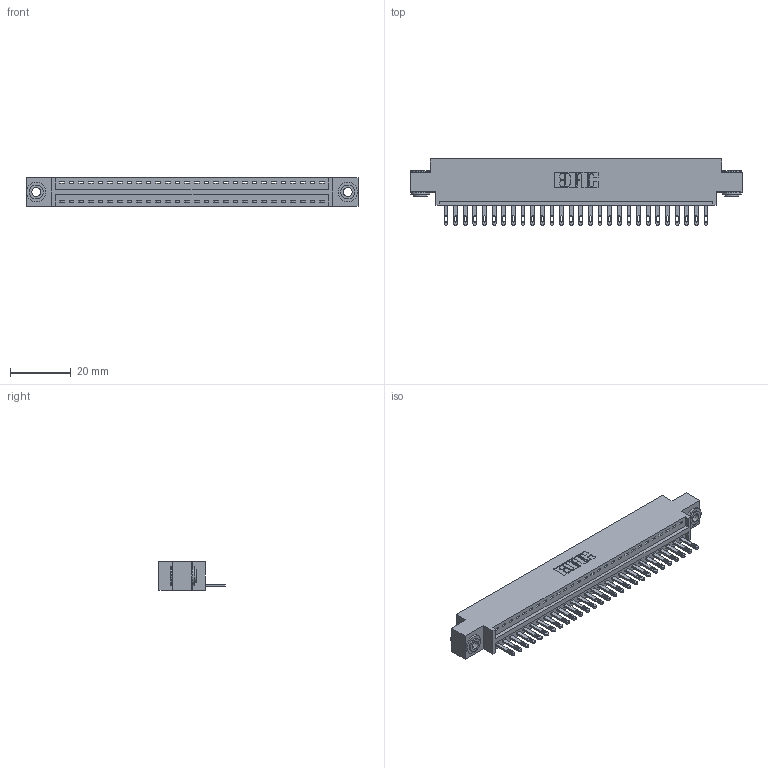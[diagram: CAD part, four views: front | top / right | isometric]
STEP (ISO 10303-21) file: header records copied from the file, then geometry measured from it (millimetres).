
FILE_DESCRIPTION (( 'STEP AP203' ), '1' );
FILE_NAME ('896-028-500-603.STEP', '2021-07-27T18:23:49', ( '' ), ( '' ), 'SwSTEP 2.0', 'SolidWorks 2020', '' );
FILE_SCHEMA (( 'CONFIG_CONTROL_DESIGN' ));
Length unit declared in the file: inch
Products named in the file (4): 345-250-002_345-250-002-102; 846 Part_0.170 Offset - 0.156 Dia-TH; 896-028-500-603; 345-292-001_345-293-100
Assembly tree (31 placements, depth 2):
  896-028-500-603
    846 Part_0.170 Offset - 0.156 Dia-TH
    345-292-001_345-293-100  x28
    345-250-002_345-250-002-102  x2
Bounding box: 109.47 x 21.84 x 9.4 mm (x, y, z)
Volume: 10264.7 mm3; surface area: 13123.3 mm2
Topology: 31 solids, 31 shells, 1676 faces, 5121 edges, 3410 vertices
Faces by surface type: plane 1042, cylinder 626, cone 8
Entity records: 19974 total; most frequent: CARTESIAN_POINT 3407, ORIENTED_EDGE 3362, DIRECTION 3055, EDGE_CURVE 1681, VECTOR 1409, LINE 1409, VERTEX_POINT 1118, AXIS2_PLACEMENT_3D 823
